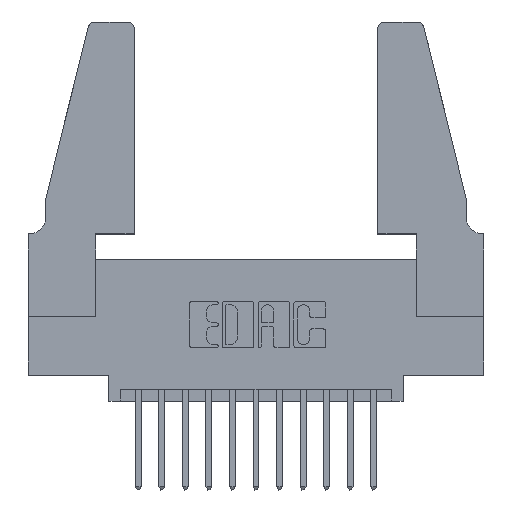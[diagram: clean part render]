
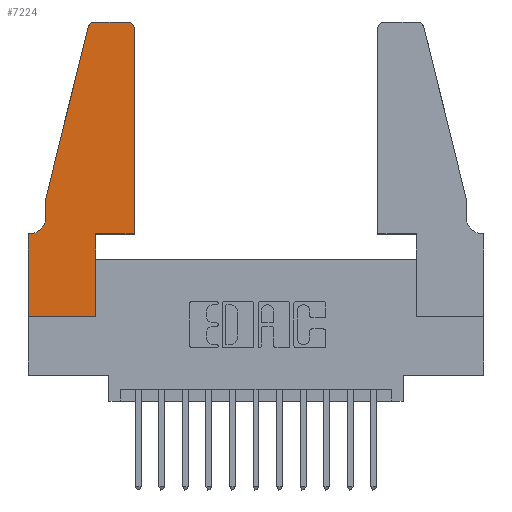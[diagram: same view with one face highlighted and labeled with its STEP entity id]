
A CAD part, top view. The second image highlights one B-rep face of the part: STEP entity #7224.
In plain terms, the highlighted planar face has unit normal (0, 0, 1).
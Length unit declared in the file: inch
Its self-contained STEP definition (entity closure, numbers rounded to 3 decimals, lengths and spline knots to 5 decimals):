
#17 = VERTEX_POINT ( 'NONE', #2323 ) ;
#203 = ORIENTED_EDGE ( 'NONE', *, *, #6616, .T. ) ;
#309 = DIRECTION ( 'NONE',  ( 0., -1., 0. ) ) ;
#439 = PLANE ( 'NONE',  #6308 ) ;
#487 = VERTEX_POINT ( 'NONE', #10182 ) ;
#698 = DIRECTION ( 'NONE',  ( 0., 0., 1. ) ) ;
#704 = LINE ( 'NONE', #11413, #6745 ) ;
#842 = EDGE_LOOP ( 'NONE', ( #2929, #6608, #5553, #4500, #1998, #9885, #12564, #203, #2949, #14323, #1662, #7200 ) ) ;
#861 = CIRCLE ( 'NONE', #1018, 0.07 ) ;
#1018 = AXIS2_PLACEMENT_3D ( 'NONE', #12268, #5385, #13389 ) ;
#1038 = VECTOR ( 'NONE', #4236, 39.37008 ) ;
#1662 = ORIENTED_EDGE ( 'NONE', *, *, #12222, .T. ) ;
#1790 = LINE ( 'NONE', #5105, #10801 ) ;
#1998 = ORIENTED_EDGE ( 'NONE', *, *, #3144, .T. ) ;
#2042 = AXIS2_PLACEMENT_3D ( 'NONE', #7892, #698, #9019 ) ;
#2323 = CARTESIAN_POINT ( 'NONE',  ( 0., 0.35, 0.37 ) ) ;
#2441 = VERTEX_POINT ( 'NONE', #7306 ) ;
#2556 = VERTEX_POINT ( 'NONE', #5069 ) ;
#2703 = FACE_OUTER_BOUND ( 'NONE', #842, .T. ) ;
#2929 = ORIENTED_EDGE ( 'NONE', *, *, #3725, .T. ) ;
#2949 = ORIENTED_EDGE ( 'NONE', *, *, #7863, .T. ) ;
#3120 = CARTESIAN_POINT ( 'NONE',  ( 0.4205, 1.25, 0.37 ) ) ;
#3144 = EDGE_CURVE ( 'NONE', #5596, #6947, #861, .T. ) ;
#3725 = EDGE_CURVE ( 'NONE', #11432, #10347, #1790, .T. ) ;
#3899 = DIRECTION ( 'NONE',  ( -1., 0., 0. ) ) ;
#3980 = EDGE_CURVE ( 'NONE', #8056, #11432, #5179, .T. ) ;
#4236 = DIRECTION ( 'NONE',  ( 1., 0., 0. ) ) ;
#4332 = CIRCLE ( 'NONE', #12765, 0.03 ) ;
#4458 = DIRECTION ( 'NONE',  ( -1., 0., 0. ) ) ;
#4500 = ORIENTED_EDGE ( 'NONE', *, *, #7782, .T. ) ;
#4637 = DIRECTION ( 'NONE',  ( 0., 0., 1. ) ) ;
#4766 = VECTOR ( 'NONE', #10064, 39.37008 ) ;
#4815 = CARTESIAN_POINT ( 'NONE',  ( 0.0055, 0.35, 0.37 ) ) ;
#5069 = CARTESIAN_POINT ( 'NONE',  ( 0.0755, 0.5, 0.37 ) ) ;
#5105 = CARTESIAN_POINT ( 'NONE',  ( 0.2605, 1.25, 0.37 ) ) ;
#5179 = CIRCLE ( 'NONE', #2042, 0.03 ) ;
#5345 = CARTESIAN_POINT ( 'NONE',  ( 0.4505, 0.35, 0.37 ) ) ;
#5385 = DIRECTION ( 'NONE',  ( 0., 0., -1. ) ) ;
#5513 = LINE ( 'NONE', #10015, #4766 ) ;
#5553 = ORIENTED_EDGE ( 'NONE', *, *, #12894, .T. ) ;
#5596 = VERTEX_POINT ( 'NONE', #12793 ) ;
#5727 = VECTOR ( 'NONE', #7412, 39.37008 ) ;
#5864 = CARTESIAN_POINT ( 'NONE',  ( 0.4505, 0.35, 0.37 ) ) ;
#5941 = CARTESIAN_POINT ( 'NONE',  ( 0.2865, 0.35, 0.37 ) ) ;
#6308 = AXIS2_PLACEMENT_3D ( 'NONE', #12208, #14455, #7707 ) ;
#6608 = ORIENTED_EDGE ( 'NONE', *, *, #10994, .T. ) ;
#6616 = EDGE_CURVE ( 'NONE', #487, #2441, #7434, .T. ) ;
#6745 = VECTOR ( 'NONE', #4458, 39.37008 ) ;
#6947 = VERTEX_POINT ( 'NONE', #4815 ) ;
#7200 = ORIENTED_EDGE ( 'NONE', *, *, #3980, .T. ) ;
#7224 = ADVANCED_FACE ( 'NONE', ( #2703 ), #439, .T. ) ;
#7306 = CARTESIAN_POINT ( 'NONE',  ( 0.2865, 0., 0.37 ) ) ;
#7412 = DIRECTION ( 'NONE',  ( 0., -1., 0. ) ) ;
#7434 = LINE ( 'NONE', #14521, #1038 ) ;
#7534 = CARTESIAN_POINT ( 'NONE',  ( 0.0755, 0.5, 0.37 ) ) ;
#7579 = LINE ( 'NONE', #7534, #13601 ) ;
#7707 = DIRECTION ( 'NONE',  ( 1., 0., 0. ) ) ;
#7782 = EDGE_CURVE ( 'NONE', #2556, #5596, #7579, .T. ) ;
#7863 = EDGE_CURVE ( 'NONE', #2441, #11873, #9165, .T. ) ;
#7892 = CARTESIAN_POINT ( 'NONE',  ( 0.4205, 1.22, 0.37 ) ) ;
#7939 = CARTESIAN_POINT ( 'NONE',  ( 0.25487, 1.22718, 0.37 ) ) ;
#8056 = VERTEX_POINT ( 'NONE', #12530 ) ;
#8261 = LINE ( 'NONE', #5345, #10916 ) ;
#8282 = DIRECTION ( 'NONE',  ( 1., 0., 0. ) ) ;
#8351 = EDGE_CURVE ( 'NONE', #17, #487, #9154, .T. ) ;
#8814 = DIRECTION ( 'NONE',  ( 0., 1., 0. ) ) ;
#9019 = DIRECTION ( 'NONE',  ( 1., 0., 0. ) ) ;
#9154 = LINE ( 'NONE', #14174, #5727 ) ;
#9165 = LINE ( 'NONE', #14439, #11848 ) ;
#9526 = VERTEX_POINT ( 'NONE', #7939 ) ;
#9581 = VECTOR ( 'NONE', #8282, 39.37008 ) ;
#9885 = ORIENTED_EDGE ( 'NONE', *, *, #11478, .T. ) ;
#9942 = LINE ( 'NONE', #13914, #9581 ) ;
#10015 = CARTESIAN_POINT ( 'NONE',  ( 0.0755, 0.5, 0.37 ) ) ;
#10064 = DIRECTION ( 'NONE',  ( -0.239, -0.971, 0. ) ) ;
#10182 = CARTESIAN_POINT ( 'NONE',  ( 0., 0., 0.37 ) ) ;
#10347 = VERTEX_POINT ( 'NONE', #11597 ) ;
#10801 = VECTOR ( 'NONE', #3899, 39.37008 ) ;
#10916 = VECTOR ( 'NONE', #11103, 39.37008 ) ;
#10994 = EDGE_CURVE ( 'NONE', #10347, #9526, #4332, .T. ) ;
#11103 = DIRECTION ( 'NONE',  ( 0., 1., 0. ) ) ;
#11413 = CARTESIAN_POINT ( 'NONE',  ( 0.0755, 0.35, 0.37 ) ) ;
#11432 = VERTEX_POINT ( 'NONE', #3120 ) ;
#11478 = EDGE_CURVE ( 'NONE', #6947, #17, #704, .T. ) ;
#11572 = CARTESIAN_POINT ( 'NONE',  ( 0.284, 1.22, 0.37 ) ) ;
#11597 = CARTESIAN_POINT ( 'NONE',  ( 0.284, 1.25, 0.37 ) ) ;
#11680 = EDGE_CURVE ( 'NONE', #11873, #14930, #9942, .T. ) ;
#11848 = VECTOR ( 'NONE', #8814, 39.37008 ) ;
#11873 = VERTEX_POINT ( 'NONE', #5941 ) ;
#12208 = CARTESIAN_POINT ( 'NONE',  ( 0., 0.35, 0.37 ) ) ;
#12222 = EDGE_CURVE ( 'NONE', #14930, #8056, #8261, .T. ) ;
#12268 = CARTESIAN_POINT ( 'NONE',  ( 0.0055, 0.42, 0.37 ) ) ;
#12530 = CARTESIAN_POINT ( 'NONE',  ( 0.4505, 1.22, 0.37 ) ) ;
#12564 = ORIENTED_EDGE ( 'NONE', *, *, #8351, .T. ) ;
#12695 = DIRECTION ( 'NONE',  ( 1., 0., 0. ) ) ;
#12765 = AXIS2_PLACEMENT_3D ( 'NONE', #11572, #4637, #12695 ) ;
#12793 = CARTESIAN_POINT ( 'NONE',  ( 0.0755, 0.42, 0.37 ) ) ;
#12894 = EDGE_CURVE ( 'NONE', #9526, #2556, #5513, .T. ) ;
#13389 = DIRECTION ( 'NONE',  ( -1., 0., 0. ) ) ;
#13601 = VECTOR ( 'NONE', #309, 39.37008 ) ;
#13914 = CARTESIAN_POINT ( 'NONE',  ( 0.4505, 0.35, 0.37 ) ) ;
#14174 = CARTESIAN_POINT ( 'NONE',  ( 0., 0., 0.37 ) ) ;
#14323 = ORIENTED_EDGE ( 'NONE', *, *, #11680, .T. ) ;
#14439 = CARTESIAN_POINT ( 'NONE',  ( 0.2865, 0.35, 0.37 ) ) ;
#14455 = DIRECTION ( 'NONE',  ( 0., 0., 1. ) ) ;
#14521 = CARTESIAN_POINT ( 'NONE',  ( 0., 0., 0.37 ) ) ;
#14930 = VERTEX_POINT ( 'NONE', #5864 ) ;
